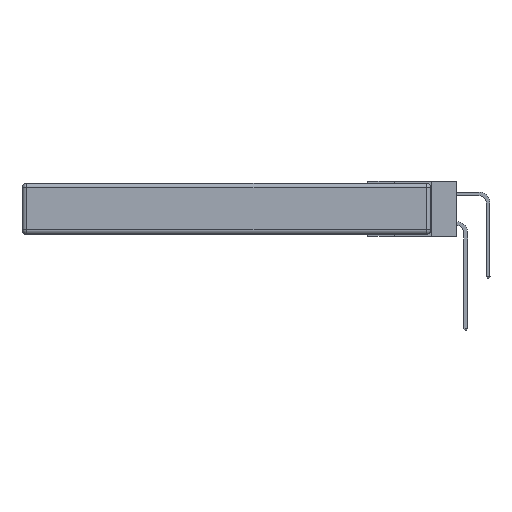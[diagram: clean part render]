
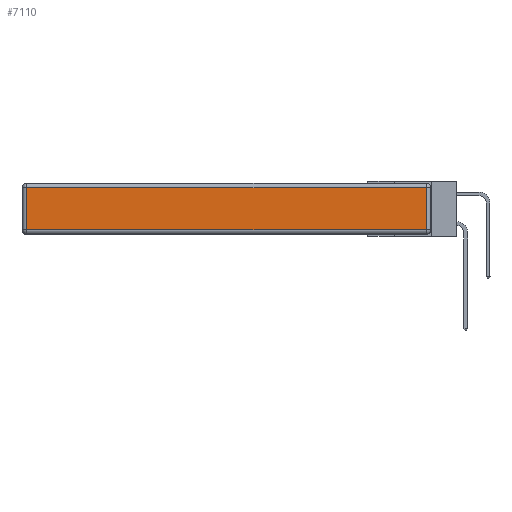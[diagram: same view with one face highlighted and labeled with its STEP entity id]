
A CAD part, left-side view. The second image highlights one B-rep face of the part: STEP entity #7110.
In plain terms, the highlighted planar face has unit normal (-1, 0, 0).
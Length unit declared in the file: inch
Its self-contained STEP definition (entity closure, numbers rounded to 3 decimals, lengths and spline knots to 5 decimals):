
#40 = VERTEX_POINT ( 'NONE', #12187 ) ;
#129 = EDGE_LOOP ( 'NONE', ( #18481, #10991, #17920, #7724 ) ) ;
#201 = LINE ( 'NONE', #2150, #5885 ) ;
#366 = EDGE_CURVE ( 'NONE', #2393, #1853, #18342, .T. ) ;
#600 = DIRECTION ( 'NONE',  ( 0., 0., -1. ) ) ;
#665 = PLANE ( 'NONE',  #20380 ) ;
#1422 = VECTOR ( 'NONE', #14215, 39.37008 ) ;
#1853 = VERTEX_POINT ( 'NONE', #5390 ) ;
#2150 = CARTESIAN_POINT ( 'NONE',  ( 0., 2.72, -0.343 ) ) ;
#2393 = VERTEX_POINT ( 'NONE', #4669 ) ;
#3129 = EDGE_CURVE ( 'NONE', #10152, #40, #3670, .T. ) ;
#3237 = CARTESIAN_POINT ( 'NONE',  ( 0., 2.75, -0.03 ) ) ;
#3398 = CARTESIAN_POINT ( 'NONE',  ( 0., 0.03, -0.343 ) ) ;
#3670 = LINE ( 'NONE', #9734, #1422 ) ;
#3880 = DIRECTION ( 'NONE',  ( 0., 0., 1. ) ) ;
#4248 = VECTOR ( 'NONE', #16130, 39.37008 ) ;
#4669 = CARTESIAN_POINT ( 'NONE',  ( 0., 0.03, -0.03 ) ) ;
#5390 = CARTESIAN_POINT ( 'NONE',  ( 0., 2.72, -0.03 ) ) ;
#5885 = VECTOR ( 'NONE', #600, 39.37008 ) ;
#6867 = EDGE_CURVE ( 'NONE', #40, #2393, #19083, .T. ) ;
#7110 = ADVANCED_FACE ( 'NONE', ( #11116 ), #665, .T. ) ;
#7724 = ORIENTED_EDGE ( 'NONE', *, *, #9691, .T. ) ;
#9669 = VECTOR ( 'NONE', #9720, 39.37008 ) ;
#9691 = EDGE_CURVE ( 'NONE', #1853, #10152, #201, .T. ) ;
#9720 = DIRECTION ( 'NONE',  ( 0., 0., 1. ) ) ;
#9734 = CARTESIAN_POINT ( 'NONE',  ( 0., 0., -0.313 ) ) ;
#10152 = VERTEX_POINT ( 'NONE', #15646 ) ;
#10991 = ORIENTED_EDGE ( 'NONE', *, *, #6867, .T. ) ;
#11116 = FACE_OUTER_BOUND ( 'NONE', #129, .T. ) ;
#11649 = DIRECTION ( 'NONE',  ( -1., 0., 0. ) ) ;
#12187 = CARTESIAN_POINT ( 'NONE',  ( 0., 0.03, -0.313 ) ) ;
#13201 = CARTESIAN_POINT ( 'NONE',  ( 0., 0., -0.343 ) ) ;
#14215 = DIRECTION ( 'NONE',  ( 0., -1., 0. ) ) ;
#15646 = CARTESIAN_POINT ( 'NONE',  ( 0., 2.72, -0.313 ) ) ;
#16130 = DIRECTION ( 'NONE',  ( 0., 1., 0. ) ) ;
#17920 = ORIENTED_EDGE ( 'NONE', *, *, #366, .T. ) ;
#18342 = LINE ( 'NONE', #3237, #4248 ) ;
#18481 = ORIENTED_EDGE ( 'NONE', *, *, #3129, .T. ) ;
#19083 = LINE ( 'NONE', #3398, #9669 ) ;
#20380 = AXIS2_PLACEMENT_3D ( 'NONE', #13201, #11649, #3880 ) ;
